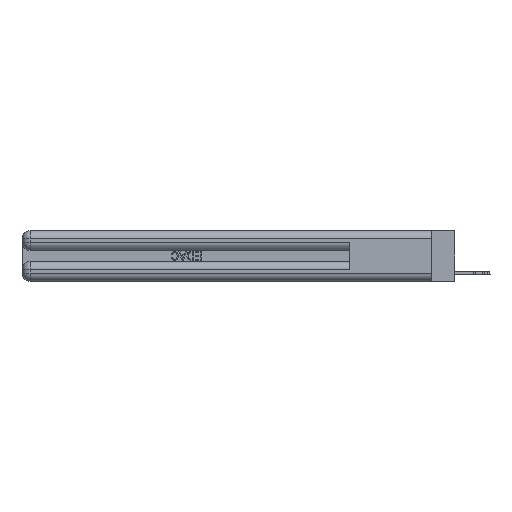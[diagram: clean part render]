
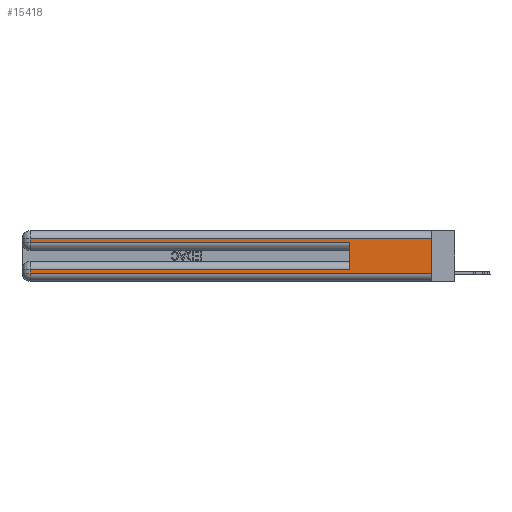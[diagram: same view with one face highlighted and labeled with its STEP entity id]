
A CAD part, left-side view. The second image highlights one B-rep face of the part: STEP entity #15418.
In plain terms, the highlighted planar face has unit normal (-1, 0, 0).
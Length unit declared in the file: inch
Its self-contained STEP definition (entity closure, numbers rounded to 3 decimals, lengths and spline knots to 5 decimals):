
#584 = EDGE_LOOP ( 'NONE', ( #19424, #25265, #24189, #16620, #27250, #5852, #7478, #11002 ) ) ;
#667 = CARTESIAN_POINT ( 'NONE',  ( 0., 2.94, 0.37 ) ) ;
#712 = CARTESIAN_POINT ( 'NONE',  ( 0., 0.6, 0.285 ) ) ;
#724 = VERTEX_POINT ( 'NONE', #10007 ) ;
#3006 = VERTEX_POINT ( 'NONE', #14891 ) ;
#3301 = EDGE_CURVE ( 'NONE', #6016, #3006, #26309, .T. ) ;
#3323 = VERTEX_POINT ( 'NONE', #712 ) ;
#5852 = ORIENTED_EDGE ( 'NONE', *, *, #20880, .T. ) ;
#6016 = VERTEX_POINT ( 'NONE', #12333 ) ;
#6316 = VERTEX_POINT ( 'NONE', #17408 ) ;
#6515 = DIRECTION ( 'NONE',  ( 0., -1., 0. ) ) ;
#6997 = LINE ( 'NONE', #25091, #23322 ) ;
#7014 = CARTESIAN_POINT ( 'NONE',  ( 0., 0., 0.085 ) ) ;
#7478 = ORIENTED_EDGE ( 'NONE', *, *, #25973, .T. ) ;
#8123 = FACE_OUTER_BOUND ( 'NONE', #584, .T. ) ;
#8315 = VECTOR ( 'NONE', #14531, 39.37008 ) ;
#8917 = CARTESIAN_POINT ( 'NONE',  ( 0., 2.94, 0.37 ) ) ;
#9516 = CARTESIAN_POINT ( 'NONE',  ( 0., 2.94, 0.285 ) ) ;
#10007 = CARTESIAN_POINT ( 'NONE',  ( 0., 0., 0.31 ) ) ;
#10457 = LINE ( 'NONE', #31740, #24812 ) ;
#10738 = VECTOR ( 'NONE', #6515, 39.37008 ) ;
#11002 = ORIENTED_EDGE ( 'NONE', *, *, #3301, .T. ) ;
#11118 = DIRECTION ( 'NONE',  ( 0., 0., 1. ) ) ;
#12045 = DIRECTION ( 'NONE',  ( 1., 0., 0. ) ) ;
#12052 = VECTOR ( 'NONE', #21680, 39.37008 ) ;
#12333 = CARTESIAN_POINT ( 'NONE',  ( 0., 2.94, 0.06 ) ) ;
#12487 = LINE ( 'NONE', #7014, #8315 ) ;
#12643 = EDGE_CURVE ( 'NONE', #25518, #3323, #29886, .T. ) ;
#13462 = LINE ( 'NONE', #667, #32354 ) ;
#14531 = DIRECTION ( 'NONE',  ( 0., 1., 0. ) ) ;
#14891 = CARTESIAN_POINT ( 'NONE',  ( 0., 0., 0.06 ) ) ;
#15418 = ADVANCED_FACE ( 'NONE', ( #8123 ), #18539, .F. ) ;
#15493 = CARTESIAN_POINT ( 'NONE',  ( 0., 0., 0.31 ) ) ;
#16398 = CARTESIAN_POINT ( 'NONE',  ( 0., 0., 0.06 ) ) ;
#16620 = ORIENTED_EDGE ( 'NONE', *, *, #12643, .T. ) ;
#17248 = CARTESIAN_POINT ( 'NONE',  ( 0., 0.6, 0.085 ) ) ;
#17408 = CARTESIAN_POINT ( 'NONE',  ( 0., 2.94, 0.31 ) ) ;
#17448 = VERTEX_POINT ( 'NONE', #19549 ) ;
#18539 = PLANE ( 'NONE',  #31539 ) ;
#18564 = EDGE_CURVE ( 'NONE', #724, #6316, #29298, .T. ) ;
#19321 = LINE ( 'NONE', #8917, #23766 ) ;
#19424 = ORIENTED_EDGE ( 'NONE', *, *, #31640, .F. ) ;
#19549 = CARTESIAN_POINT ( 'NONE',  ( 0., 2.94, 0.085 ) ) ;
#20880 = EDGE_CURVE ( 'NONE', #25009, #17448, #12487, .T. ) ;
#21680 = DIRECTION ( 'NONE',  ( 0., -1., 0. ) ) ;
#22704 = DIRECTION ( 'NONE',  ( 0., 0., -1. ) ) ;
#23322 = VECTOR ( 'NONE', #22704, 39.37008 ) ;
#23766 = VECTOR ( 'NONE', #29070, 39.37008 ) ;
#23818 = CARTESIAN_POINT ( 'NONE',  ( 0., 0., 0.37 ) ) ;
#24020 = DIRECTION ( 'NONE',  ( 0., 0., -1. ) ) ;
#24189 = ORIENTED_EDGE ( 'NONE', *, *, #29734, .T. ) ;
#24812 = VECTOR ( 'NONE', #11118, 39.37008 ) ;
#25009 = VERTEX_POINT ( 'NONE', #17248 ) ;
#25091 = CARTESIAN_POINT ( 'NONE',  ( 0., 0., 0.37 ) ) ;
#25173 = DIRECTION ( 'NONE',  ( 0., 0., -1. ) ) ;
#25265 = ORIENTED_EDGE ( 'NONE', *, *, #18564, .T. ) ;
#25518 = VERTEX_POINT ( 'NONE', #9516 ) ;
#25915 = DIRECTION ( 'NONE',  ( 0., 1., 0. ) ) ;
#25973 = EDGE_CURVE ( 'NONE', #17448, #6016, #13462, .T. ) ;
#26309 = LINE ( 'NONE', #16398, #12052 ) ;
#27242 = EDGE_CURVE ( 'NONE', #25009, #3323, #10457, .T. ) ;
#27250 = ORIENTED_EDGE ( 'NONE', *, *, #27242, .F. ) ;
#27510 = CARTESIAN_POINT ( 'NONE',  ( 0., 0., 0.285 ) ) ;
#27812 = VECTOR ( 'NONE', #25915, 39.37008 ) ;
#29070 = DIRECTION ( 'NONE',  ( 0., 0., -1. ) ) ;
#29298 = LINE ( 'NONE', #15493, #27812 ) ;
#29734 = EDGE_CURVE ( 'NONE', #6316, #25518, #19321, .T. ) ;
#29886 = LINE ( 'NONE', #27510, #10738 ) ;
#31539 = AXIS2_PLACEMENT_3D ( 'NONE', #23818, #12045, #25173 ) ;
#31640 = EDGE_CURVE ( 'NONE', #724, #3006, #6997, .T. ) ;
#31740 = CARTESIAN_POINT ( 'NONE',  ( 0., 0.6, 0.145 ) ) ;
#32354 = VECTOR ( 'NONE', #24020, 39.37008 ) ;
